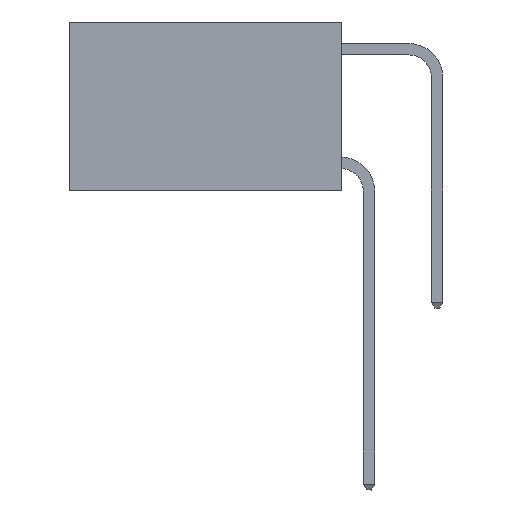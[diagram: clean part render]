
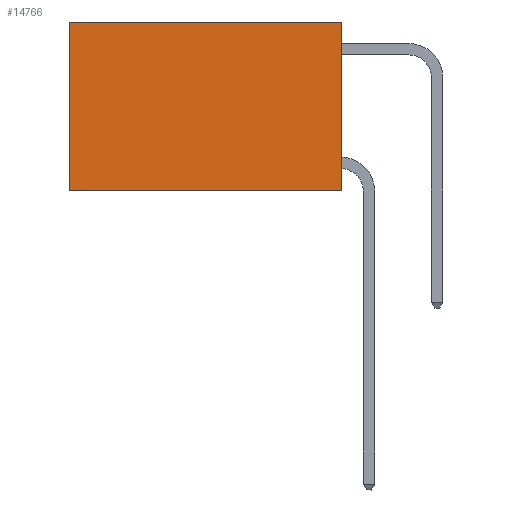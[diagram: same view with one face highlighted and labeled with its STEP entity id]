
A CAD part, left-side view. The second image highlights one B-rep face of the part: STEP entity #14766.
In plain terms, the highlighted planar face has unit normal (-1, 0, 0).
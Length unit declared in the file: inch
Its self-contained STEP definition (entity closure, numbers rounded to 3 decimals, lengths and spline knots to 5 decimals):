
#22 = EDGE_CURVE ( 'NONE', #12780, #18311, #15774, .T. ) ;
#386 = ORIENTED_EDGE ( 'NONE', *, *, #6401, .T. ) ;
#1474 = PLANE ( 'NONE',  #1535 ) ;
#1535 = AXIS2_PLACEMENT_3D ( 'NONE', #11543, #2979, #12958 ) ;
#1751 = CARTESIAN_POINT ( 'NONE',  ( 0.2625, 0., 0. ) ) ;
#1797 = VECTOR ( 'NONE', #15174, 39.37008 ) ;
#1933 = DIRECTION ( 'NONE',  ( 0., 1., 0. ) ) ;
#2262 = LINE ( 'NONE', #18037, #1797 ) ;
#2382 = EDGE_CURVE ( 'NONE', #8604, #18311, #9315, .T. ) ;
#2409 = VERTEX_POINT ( 'NONE', #16022 ) ;
#2624 = CARTESIAN_POINT ( 'NONE',  ( 0.2625, 0.6, -0.37 ) ) ;
#2880 = VECTOR ( 'NONE', #3315, 39.37008 ) ;
#2979 = DIRECTION ( 'NONE',  ( 1., 0., 0. ) ) ;
#3315 = DIRECTION ( 'NONE',  ( 0., 1., 0. ) ) ;
#3351 = ORIENTED_EDGE ( 'NONE', *, *, #11244, .F. ) ;
#3898 = CARTESIAN_POINT ( 'NONE',  ( 0.2625, 0., -0.37 ) ) ;
#6401 = EDGE_CURVE ( 'NONE', #2409, #8604, #17597, .T. ) ;
#7288 = CARTESIAN_POINT ( 'NONE',  ( 0.2625, 0., -0.37 ) ) ;
#8323 = ORIENTED_EDGE ( 'NONE', *, *, #2382, .T. ) ;
#8604 = VERTEX_POINT ( 'NONE', #18361 ) ;
#9315 = LINE ( 'NONE', #16470, #16382 ) ;
#11244 = EDGE_CURVE ( 'NONE', #2409, #12780, #2262, .T. ) ;
#11543 = CARTESIAN_POINT ( 'NONE',  ( 0.2625, 0., 0. ) ) ;
#11995 = FACE_OUTER_BOUND ( 'NONE', #17584, .T. ) ;
#12009 = VECTOR ( 'NONE', #1933, 39.37008 ) ;
#12780 = VERTEX_POINT ( 'NONE', #7288 ) ;
#12958 = DIRECTION ( 'NONE',  ( 0., 0., -1. ) ) ;
#14766 = ADVANCED_FACE ( 'NONE', ( #11995 ), #1474, .F. ) ;
#15174 = DIRECTION ( 'NONE',  ( 0., 0., -1. ) ) ;
#15774 = LINE ( 'NONE', #3898, #12009 ) ;
#16022 = CARTESIAN_POINT ( 'NONE',  ( 0.2625, 0., 0. ) ) ;
#16382 = VECTOR ( 'NONE', #16392, 39.37008 ) ;
#16392 = DIRECTION ( 'NONE',  ( 0., 0., -1. ) ) ;
#16394 = ORIENTED_EDGE ( 'NONE', *, *, #22, .F. ) ;
#16470 = CARTESIAN_POINT ( 'NONE',  ( 0.2625, 0.6, 0. ) ) ;
#17584 = EDGE_LOOP ( 'NONE', ( #8323, #16394, #3351, #386 ) ) ;
#17597 = LINE ( 'NONE', #1751, #2880 ) ;
#18037 = CARTESIAN_POINT ( 'NONE',  ( 0.2625, 0., 0. ) ) ;
#18311 = VERTEX_POINT ( 'NONE', #2624 ) ;
#18361 = CARTESIAN_POINT ( 'NONE',  ( 0.2625, 0.6, 0. ) ) ;
